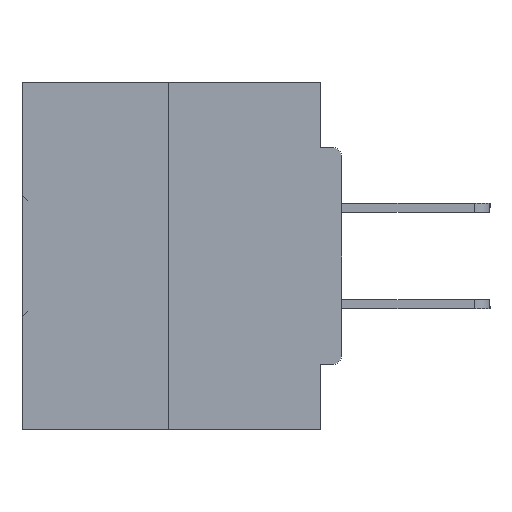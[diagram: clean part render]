
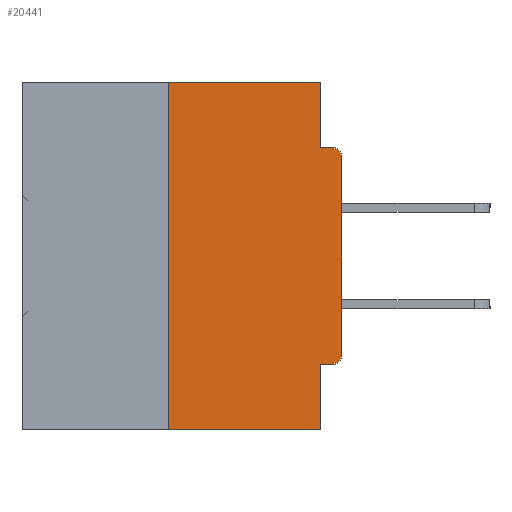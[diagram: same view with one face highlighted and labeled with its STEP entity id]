
A CAD part, left-side view. The second image highlights one B-rep face of the part: STEP entity #20441.
In plain terms, the highlighted planar face has unit normal (-1, 0, 0).
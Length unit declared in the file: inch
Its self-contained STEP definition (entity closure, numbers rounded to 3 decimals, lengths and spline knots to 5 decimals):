
#1083 = EDGE_CURVE ( 'NONE', #37242, #10105, #45582, .T. ) ;
#1647 = EDGE_CURVE ( 'NONE', #29724, #10105, #17880, .T. ) ;
#3471 = VERTEX_POINT ( 'NONE', #39857 ) ;
#3476 = FACE_OUTER_BOUND ( 'NONE', #5102, .T. ) ;
#3868 = LINE ( 'NONE', #40777, #24236 ) ;
#5102 = EDGE_LOOP ( 'NONE', ( #42280, #7773, #23179, #44563, #35822, #31639, #5266, #25547, #37320, #20873 ) ) ;
#5266 = ORIENTED_EDGE ( 'NONE', *, *, #16977, .T. ) ;
#5340 = CARTESIAN_POINT ( 'NONE',  ( 0., 0., -0.1085 ) ) ;
#5343 = CARTESIAN_POINT ( 'NONE',  ( 0., 0., -0.0935 ) ) ;
#5797 = VECTOR ( 'NONE', #39193, 39.37008 ) ;
#6667 = CARTESIAN_POINT ( 'NONE',  ( 0., 0.031, 0. ) ) ;
#7049 = VECTOR ( 'NONE', #34818, 39.37008 ) ;
#7187 = VERTEX_POINT ( 'NONE', #14556 ) ;
#7773 = ORIENTED_EDGE ( 'NONE', *, *, #42772, .F. ) ;
#8395 = LINE ( 'NONE', #16566, #34912 ) ;
#9814 = DIRECTION ( 'NONE',  ( 1., 0., 0. ) ) ;
#10105 = VERTEX_POINT ( 'NONE', #25802 ) ;
#10918 = VERTEX_POINT ( 'NONE', #40570 ) ;
#11214 = CARTESIAN_POINT ( 'NONE',  ( 0., 0.25, 0. ) ) ;
#11663 = VECTOR ( 'NONE', #30579, 39.37008 ) ;
#12836 = EDGE_CURVE ( 'NONE', #3471, #29820, #8395, .T. ) ;
#13893 = LINE ( 'NONE', #6667, #27442 ) ;
#13915 = DIRECTION ( 'NONE',  ( 0., 0., -1. ) ) ;
#14328 = CARTESIAN_POINT ( 'NONE',  ( 0., 0.25, -0.5 ) ) ;
#14556 = CARTESIAN_POINT ( 'NONE',  ( 0., 0., -0.3915 ) ) ;
#14973 = EDGE_CURVE ( 'NONE', #39860, #10918, #21746, .T. ) ;
#15242 = DIRECTION ( 'NONE',  ( 0., 0., -1. ) ) ;
#16206 = LINE ( 'NONE', #11214, #40410 ) ;
#16566 = CARTESIAN_POINT ( 'NONE',  ( 0., 0.46, 0. ) ) ;
#16916 = VERTEX_POINT ( 'NONE', #45296 ) ;
#16977 = EDGE_CURVE ( 'NONE', #7187, #37242, #41909, .T. ) ;
#17880 = LINE ( 'NONE', #5343, #11663 ) ;
#19126 = CARTESIAN_POINT ( 'NONE',  ( 0., 0.015, -0.1085 ) ) ;
#20441 = ADVANCED_FACE ( 'NONE', ( #3476 ), #30080, .F. ) ;
#20873 = ORIENTED_EDGE ( 'NONE', *, *, #25659, .F. ) ;
#21218 = CARTESIAN_POINT ( 'NONE',  ( 0., 0.031, -0.5 ) ) ;
#21746 = LINE ( 'NONE', #31204, #7049 ) ;
#21903 = VECTOR ( 'NONE', #28916, 39.37008 ) ;
#22049 = CARTESIAN_POINT ( 'NONE',  ( 0., 0.015, -0.3915 ) ) ;
#22317 = EDGE_CURVE ( 'NONE', #39860, #7187, #28464, .T. ) ;
#22485 = LINE ( 'NONE', #21218, #21903 ) ;
#22664 = DIRECTION ( 'NONE',  ( 0., -1., 0. ) ) ;
#22691 = AXIS2_PLACEMENT_3D ( 'NONE', #22049, #29740, #15242 ) ;
#23179 = ORIENTED_EDGE ( 'NONE', *, *, #41628, .T. ) ;
#24236 = VECTOR ( 'NONE', #22664, 39.37008 ) ;
#24606 = VERTEX_POINT ( 'NONE', #14328 ) ;
#25547 = ORIENTED_EDGE ( 'NONE', *, *, #1083, .T. ) ;
#25659 = EDGE_CURVE ( 'NONE', #29820, #29724, #13893, .T. ) ;
#25802 = CARTESIAN_POINT ( 'NONE',  ( 0., 0.015, -0.0935 ) ) ;
#26713 = DIRECTION ( 'NONE',  ( -1., 0., 0. ) ) ;
#27442 = VECTOR ( 'NONE', #13915, 39.37008 ) ;
#28464 = CIRCLE ( 'NONE', #22691, 0.015 ) ;
#28702 = CARTESIAN_POINT ( 'NONE',  ( 0., 0.015, -0.4065 ) ) ;
#28916 = DIRECTION ( 'NONE',  ( 0., 0., -1. ) ) ;
#29724 = VERTEX_POINT ( 'NONE', #36796 ) ;
#29740 = DIRECTION ( 'NONE',  ( -1., 0., 0. ) ) ;
#29820 = VERTEX_POINT ( 'NONE', #44862 ) ;
#30080 = PLANE ( 'NONE',  #30615 ) ;
#30579 = DIRECTION ( 'NONE',  ( 0., -1., 0. ) ) ;
#30615 = AXIS2_PLACEMENT_3D ( 'NONE', #42311, #9814, #41704 ) ;
#31204 = CARTESIAN_POINT ( 'NONE',  ( 0., 0., -0.4065 ) ) ;
#31639 = ORIENTED_EDGE ( 'NONE', *, *, #22317, .T. ) ;
#34818 = DIRECTION ( 'NONE',  ( 0., 1., 0. ) ) ;
#34912 = VECTOR ( 'NONE', #35286, 39.37008 ) ;
#35286 = DIRECTION ( 'NONE',  ( 0., -1., 0. ) ) ;
#35822 = ORIENTED_EDGE ( 'NONE', *, *, #14973, .F. ) ;
#35865 = CARTESIAN_POINT ( 'NONE',  ( 0., 0., 0. ) ) ;
#36796 = CARTESIAN_POINT ( 'NONE',  ( 0., 0.031, -0.0935 ) ) ;
#37242 = VERTEX_POINT ( 'NONE', #5340 ) ;
#37320 = ORIENTED_EDGE ( 'NONE', *, *, #1647, .F. ) ;
#39193 = DIRECTION ( 'NONE',  ( 0., 0., 1. ) ) ;
#39857 = CARTESIAN_POINT ( 'NONE',  ( 0., 0.25, 0. ) ) ;
#39860 = VERTEX_POINT ( 'NONE', #28702 ) ;
#40410 = VECTOR ( 'NONE', #43868, 39.37008 ) ;
#40570 = CARTESIAN_POINT ( 'NONE',  ( 0., 0.031, -0.4065 ) ) ;
#40777 = CARTESIAN_POINT ( 'NONE',  ( 0., 0.46, -0.5 ) ) ;
#41628 = EDGE_CURVE ( 'NONE', #24606, #16916, #3868, .T. ) ;
#41704 = DIRECTION ( 'NONE',  ( 0., 0., -1. ) ) ;
#41909 = LINE ( 'NONE', #35865, #5797 ) ;
#42124 = EDGE_CURVE ( 'NONE', #10918, #16916, #22485, .T. ) ;
#42280 = ORIENTED_EDGE ( 'NONE', *, *, #12836, .F. ) ;
#42311 = CARTESIAN_POINT ( 'NONE',  ( 0., 0.46, 0. ) ) ;
#42772 = EDGE_CURVE ( 'NONE', #24606, #3471, #16206, .T. ) ;
#43868 = DIRECTION ( 'NONE',  ( 0., 0., 1. ) ) ;
#44275 = AXIS2_PLACEMENT_3D ( 'NONE', #19126, #26713, #44371 ) ;
#44371 = DIRECTION ( 'NONE',  ( 0., 0., -1. ) ) ;
#44563 = ORIENTED_EDGE ( 'NONE', *, *, #42124, .F. ) ;
#44862 = CARTESIAN_POINT ( 'NONE',  ( 0., 0.031, 0. ) ) ;
#45296 = CARTESIAN_POINT ( 'NONE',  ( 0., 0.031, -0.5 ) ) ;
#45582 = CIRCLE ( 'NONE', #44275, 0.015 ) ;
